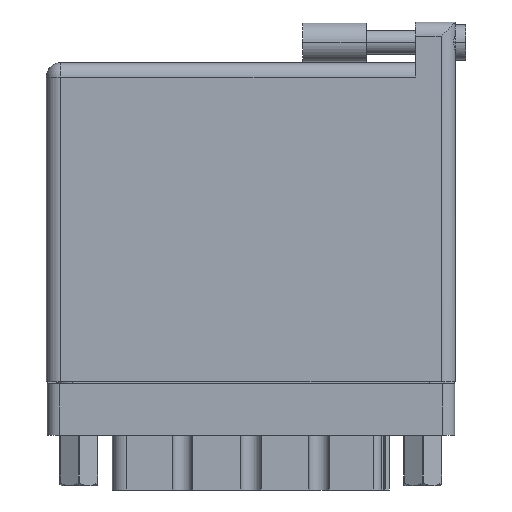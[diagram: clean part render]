
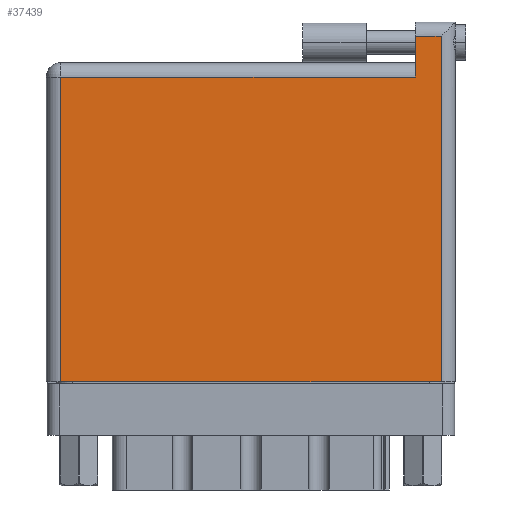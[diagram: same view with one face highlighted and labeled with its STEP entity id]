
A CAD part, front view. The second image highlights one B-rep face of the part: STEP entity #37439.
In plain terms, the highlighted face is planar.
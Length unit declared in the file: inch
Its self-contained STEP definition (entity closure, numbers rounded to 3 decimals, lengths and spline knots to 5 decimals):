
#217 = LINE ( 'NONE', #31883, #39270 ) ;
#786 = DIRECTION ( 'NONE',  ( 0., -1., 0. ) ) ;
#883 = CARTESIAN_POINT ( 'NONE',  ( 1.938, 1.696, 0. ) ) ;
#2596 = CARTESIAN_POINT ( 'NONE',  ( 0.07, 0., 0. ) ) ;
#4489 = EDGE_CURVE ( 'NONE', #7912, #48315, #13104, .T. ) ;
#4756 = ORIENTED_EDGE ( 'NONE', *, *, #39165, .T. ) ;
#5177 = ORIENTED_EDGE ( 'NONE', *, *, #24225, .T. ) ;
#6050 = CARTESIAN_POINT ( 'NONE',  ( 0.07, 0., 0. ) ) ;
#7398 = VERTEX_POINT ( 'NONE', #2596 ) ;
#7912 = VERTEX_POINT ( 'NONE', #46961 ) ;
#9496 = ORIENTED_EDGE ( 'NONE', *, *, #4489, .T. ) ;
#10299 = LINE ( 'NONE', #44548, #29554 ) ;
#10469 = VERTEX_POINT ( 'NONE', #883 ) ;
#10678 = CARTESIAN_POINT ( 'NONE',  ( 0., 1.566, 0. ) ) ;
#11634 = LINE ( 'NONE', #25718, #20573 ) ;
#11907 = CARTESIAN_POINT ( 'NONE',  ( 1.938, 0., 0. ) ) ;
#12392 = VECTOR ( 'NONE', #17535, 39.37008 ) ;
#13104 = LINE ( 'NONE', #35693, #39525 ) ;
#13206 = DIRECTION ( 'NONE',  ( -1., 0., 0. ) ) ;
#13300 = EDGE_CURVE ( 'NONE', #49099, #10469, #11634, .T. ) ;
#15526 = FACE_OUTER_BOUND ( 'NONE', #48532, .T. ) ;
#15749 = VECTOR ( 'NONE', #46364, 39.37008 ) ;
#17535 = DIRECTION ( 'NONE',  ( 0., -1., 0. ) ) ;
#18258 = DIRECTION ( 'NONE',  ( 0., 0., -1. ) ) ;
#19676 = EDGE_CURVE ( 'NONE', #20136, #7398, #23211, .T. ) ;
#20063 = CARTESIAN_POINT ( 'NONE',  ( 1.811, 1.496, 0. ) ) ;
#20136 = VERTEX_POINT ( 'NONE', #24032 ) ;
#20196 = ORIENTED_EDGE ( 'NONE', *, *, #13300, .T. ) ;
#20573 = VECTOR ( 'NONE', #41453, 39.37008 ) ;
#21131 = AXIS2_PLACEMENT_3D ( 'NONE', #10678, #18258, #33671 ) ;
#23211 = LINE ( 'NONE', #6050, #12392 ) ;
#24032 = CARTESIAN_POINT ( 'NONE',  ( 0.07, 1.496, 0. ) ) ;
#24225 = EDGE_CURVE ( 'NONE', #48315, #20136, #217, .T. ) ;
#25718 = CARTESIAN_POINT ( 'NONE',  ( 1.938, 1.766, 0. ) ) ;
#29554 = VECTOR ( 'NONE', #13206, 39.37008 ) ;
#31883 = CARTESIAN_POINT ( 'NONE',  ( 0., 1.496, 0. ) ) ;
#33671 = DIRECTION ( 'NONE',  ( -1., 0., 0. ) ) ;
#34024 = EDGE_CURVE ( 'NONE', #7398, #49099, #43973, .T. ) ;
#35693 = CARTESIAN_POINT ( 'NONE',  ( 1.811, 1.766, 0. ) ) ;
#37439 = ADVANCED_FACE ( 'NONE', ( #15526 ), #40554, .F. ) ;
#39165 = EDGE_CURVE ( 'NONE', #10469, #7912, #10299, .T. ) ;
#39270 = VECTOR ( 'NONE', #42947, 39.37008 ) ;
#39525 = VECTOR ( 'NONE', #786, 39.37008 ) ;
#40554 = PLANE ( 'NONE',  #21131 ) ;
#41453 = DIRECTION ( 'NONE',  ( 0., 1., 0. ) ) ;
#41798 = ORIENTED_EDGE ( 'NONE', *, *, #34024, .T. ) ;
#42524 = CARTESIAN_POINT ( 'NONE',  ( 0., 0., 0. ) ) ;
#42947 = DIRECTION ( 'NONE',  ( -1., 0., 0. ) ) ;
#43973 = LINE ( 'NONE', #42524, #15749 ) ;
#44548 = CARTESIAN_POINT ( 'NONE',  ( 0., 1.696, 0. ) ) ;
#46364 = DIRECTION ( 'NONE',  ( 1., 0., 0. ) ) ;
#46961 = CARTESIAN_POINT ( 'NONE',  ( 1.811, 1.696, 0. ) ) ;
#48315 = VERTEX_POINT ( 'NONE', #20063 ) ;
#48532 = EDGE_LOOP ( 'NONE', ( #41798, #20196, #4756, #9496, #5177, #48693 ) ) ;
#48693 = ORIENTED_EDGE ( 'NONE', *, *, #19676, .T. ) ;
#49099 = VERTEX_POINT ( 'NONE', #11907 ) ;
